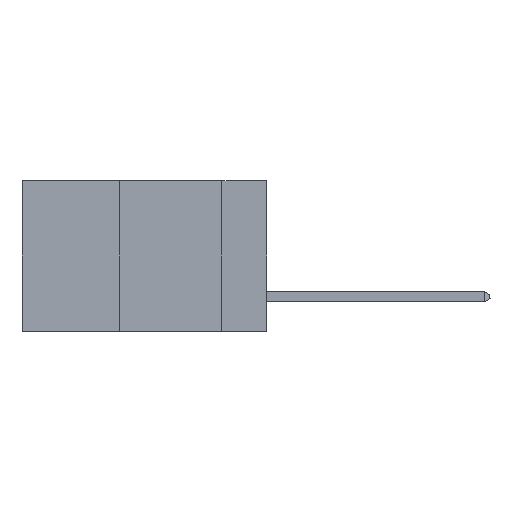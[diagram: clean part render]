
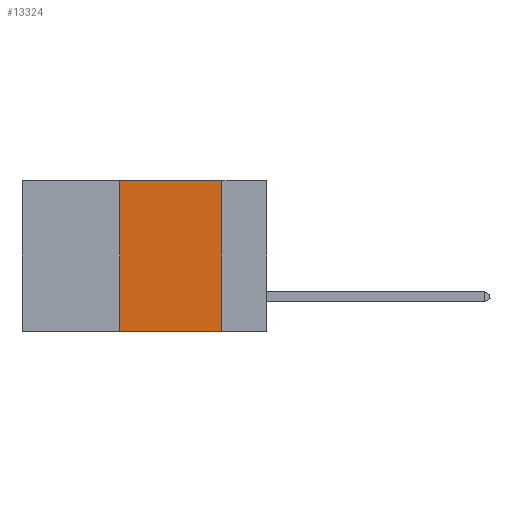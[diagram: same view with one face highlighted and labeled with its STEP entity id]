
A CAD part, left-side view. The second image highlights one B-rep face of the part: STEP entity #13324.
In plain terms, the highlighted planar face has unit normal (-1, 0, 0).
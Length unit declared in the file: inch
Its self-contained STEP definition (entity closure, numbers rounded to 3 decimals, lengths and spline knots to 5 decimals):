
#2148 = CARTESIAN_POINT ( 'NONE',  ( 0., 0.11, -0.37 ) ) ;
#2174 = CARTESIAN_POINT ( 'NONE',  ( 0., 0.6, 0. ) ) ;
#2298 = EDGE_CURVE ( 'NONE', #4252, #20320, #10602, .T. ) ;
#2534 = CARTESIAN_POINT ( 'NONE',  ( 0., 0.36, 0. ) ) ;
#2890 = VERTEX_POINT ( 'NONE', #11896 ) ;
#4252 = VERTEX_POINT ( 'NONE', #4548 ) ;
#4548 = CARTESIAN_POINT ( 'NONE',  ( 0., 0.36, -0.37 ) ) ;
#5658 = VECTOR ( 'NONE', #24896, 39.37008 ) ;
#6290 = CARTESIAN_POINT ( 'NONE',  ( 0., 0.36, 0. ) ) ;
#6507 = EDGE_CURVE ( 'NONE', #2890, #20320, #24558, .T. ) ;
#6899 = ORIENTED_EDGE ( 'NONE', *, *, #18497, .F. ) ;
#6981 = CARTESIAN_POINT ( 'NONE',  ( 0., 0.11, 0. ) ) ;
#7391 = FACE_OUTER_BOUND ( 'NONE', #17228, .T. ) ;
#8183 = ORIENTED_EDGE ( 'NONE', *, *, #18739, .F. ) ;
#8208 = DIRECTION ( 'NONE',  ( 0., 0., 1. ) ) ;
#10286 = PLANE ( 'NONE',  #11136 ) ;
#10602 = LINE ( 'NONE', #23682, #20178 ) ;
#11136 = AXIS2_PLACEMENT_3D ( 'NONE', #14208, #12214, #14379 ) ;
#11896 = CARTESIAN_POINT ( 'NONE',  ( 0., 0.11, 0. ) ) ;
#12214 = DIRECTION ( 'NONE',  ( 1., 0., 0. ) ) ;
#12573 = LINE ( 'NONE', #6290, #17059 ) ;
#13324 = ADVANCED_FACE ( 'NONE', ( #7391 ), #10286, .F. ) ;
#14045 = DIRECTION ( 'NONE',  ( 0., -1., 0. ) ) ;
#14208 = CARTESIAN_POINT ( 'NONE',  ( 0., 0.6, 0. ) ) ;
#14379 = DIRECTION ( 'NONE',  ( 0., 0., -1. ) ) ;
#16900 = DIRECTION ( 'NONE',  ( 0., 0., -1. ) ) ;
#17059 = VECTOR ( 'NONE', #8208, 39.37008 ) ;
#17228 = EDGE_LOOP ( 'NONE', ( #18858, #8183, #6899, #20783 ) ) ;
#18497 = EDGE_CURVE ( 'NONE', #4252, #20286, #12573, .T. ) ;
#18739 = EDGE_CURVE ( 'NONE', #20286, #2890, #19743, .T. ) ;
#18858 = ORIENTED_EDGE ( 'NONE', *, *, #6507, .F. ) ;
#19707 = VECTOR ( 'NONE', #16900, 39.37008 ) ;
#19743 = LINE ( 'NONE', #2174, #5658 ) ;
#20178 = VECTOR ( 'NONE', #14045, 39.37008 ) ;
#20286 = VERTEX_POINT ( 'NONE', #2534 ) ;
#20320 = VERTEX_POINT ( 'NONE', #2148 ) ;
#20783 = ORIENTED_EDGE ( 'NONE', *, *, #2298, .T. ) ;
#23682 = CARTESIAN_POINT ( 'NONE',  ( 0., 0.6, -0.37 ) ) ;
#24558 = LINE ( 'NONE', #6981, #19707 ) ;
#24896 = DIRECTION ( 'NONE',  ( 0., -1., 0. ) ) ;
